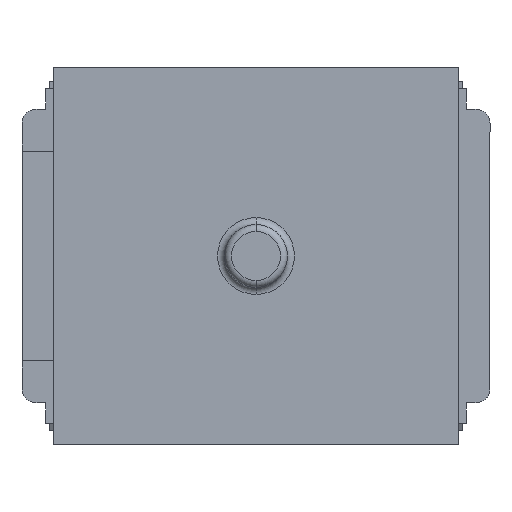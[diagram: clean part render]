
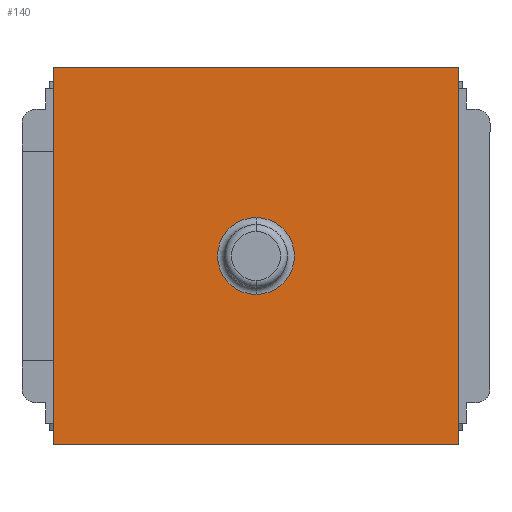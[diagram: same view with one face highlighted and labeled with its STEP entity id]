
A CAD part, front view. The second image highlights one B-rep face of the part: STEP entity #140.
In plain terms, the highlighted planar face has unit normal (0, -1, 0).
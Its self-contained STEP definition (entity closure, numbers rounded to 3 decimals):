
#29 = CARTESIAN_POINT ( 'NONE',  ( -14.5, 0., 13.5 ) ) ;
#38 = VERTEX_POINT ( 'NONE', #10297 ) ;
#67 = DIRECTION ( 'NONE',  ( 0., -1., 0. ) ) ;
#140 = ADVANCED_FACE ( 'NONE', ( #1272, #4230 ), #11520, .T. ) ;
#559 = LINE ( 'NONE', #11567, #11957 ) ;
#809 = LINE ( 'NONE', #8428, #12501 ) ;
#1272 = FACE_OUTER_BOUND ( 'NONE', #3683, .T. ) ;
#1480 = CARTESIAN_POINT ( 'NONE',  ( -14.5, 0., -13.5 ) ) ;
#1670 = DIRECTION ( 'NONE',  ( 0., 0., -1. ) ) ;
#1696 = DIRECTION ( 'NONE',  ( 1., 0., 0. ) ) ;
#2077 = ORIENTED_EDGE ( 'NONE', *, *, #9021, .F. ) ;
#2322 = VERTEX_POINT ( 'NONE', #12895 ) ;
#2893 = DIRECTION ( 'NONE',  ( -1., 0., 0. ) ) ;
#3023 = ORIENTED_EDGE ( 'NONE', *, *, #13638, .F. ) ;
#3104 = CARTESIAN_POINT ( 'NONE',  ( 14.5, 0., -13.5 ) ) ;
#3201 = CARTESIAN_POINT ( 'NONE',  ( 0., 0., 0. ) ) ;
#3608 = DIRECTION ( 'NONE',  ( 0., 1., 0. ) ) ;
#3683 = EDGE_LOOP ( 'NONE', ( #12785, #5862, #3023, #2077 ) ) ;
#4230 = FACE_BOUND ( 'NONE', #7990, .T. ) ;
#4301 = DIRECTION ( 'NONE',  ( 0., 0., 1. ) ) ;
#4398 = ORIENTED_EDGE ( 'NONE', *, *, #6905, .T. ) ;
#5103 = DIRECTION ( 'NONE',  ( 0., 0., 1. ) ) ;
#5650 = CIRCLE ( 'NONE', #9942, 2.75 ) ;
#5862 = ORIENTED_EDGE ( 'NONE', *, *, #6649, .F. ) ;
#6649 = EDGE_CURVE ( 'NONE', #13447, #38, #559, .T. ) ;
#6742 = VECTOR ( 'NONE', #2893, 1000. ) ;
#6905 = EDGE_CURVE ( 'NONE', #7836, #2322, #10182, .T. ) ;
#7040 = ORIENTED_EDGE ( 'NONE', *, *, #11708, .T. ) ;
#7765 = DIRECTION ( 'NONE',  ( 0., 0., -1. ) ) ;
#7836 = VERTEX_POINT ( 'NONE', #13897 ) ;
#7990 = EDGE_LOOP ( 'NONE', ( #4398, #7040 ) ) ;
#8428 = CARTESIAN_POINT ( 'NONE',  ( -14.5, 0., 13.5 ) ) ;
#8449 = AXIS2_PLACEMENT_3D ( 'NONE', #13265, #67, #7765 ) ;
#8809 = VERTEX_POINT ( 'NONE', #3104 ) ;
#9021 = EDGE_CURVE ( 'NONE', #8809, #10496, #9664, .T. ) ;
#9354 = CARTESIAN_POINT ( 'NONE',  ( 14.5, 0., 13.5 ) ) ;
#9465 = LINE ( 'NONE', #9354, #12097 ) ;
#9519 = EDGE_CURVE ( 'NONE', #38, #8809, #9465, .T. ) ;
#9664 = LINE ( 'NONE', #1480, #6742 ) ;
#9942 = AXIS2_PLACEMENT_3D ( 'NONE', #3201, #10889, #4301 ) ;
#9962 = CARTESIAN_POINT ( 'NONE',  ( -14.5, 0., -13.5 ) ) ;
#10182 = CIRCLE ( 'NONE', #13601, 2.75 ) ;
#10183 = CARTESIAN_POINT ( 'NONE',  ( 0., 0., 0. ) ) ;
#10297 = CARTESIAN_POINT ( 'NONE',  ( 14.5, 0., 13.5 ) ) ;
#10496 = VERTEX_POINT ( 'NONE', #9962 ) ;
#10889 = DIRECTION ( 'NONE',  ( 0., 1., 0. ) ) ;
#11308 = DIRECTION ( 'NONE',  ( 0., 0., 1. ) ) ;
#11520 = PLANE ( 'NONE',  #8449 ) ;
#11567 = CARTESIAN_POINT ( 'NONE',  ( -14.5, 0., 13.5 ) ) ;
#11708 = EDGE_CURVE ( 'NONE', #2322, #7836, #5650, .T. ) ;
#11957 = VECTOR ( 'NONE', #1696, 1000. ) ;
#12097 = VECTOR ( 'NONE', #1670, 1000. ) ;
#12501 = VECTOR ( 'NONE', #5103, 1000. ) ;
#12785 = ORIENTED_EDGE ( 'NONE', *, *, #9519, .F. ) ;
#12895 = CARTESIAN_POINT ( 'NONE',  ( 0., 0., 2.75 ) ) ;
#13265 = CARTESIAN_POINT ( 'NONE',  ( 0., 0., 0. ) ) ;
#13447 = VERTEX_POINT ( 'NONE', #29 ) ;
#13601 = AXIS2_PLACEMENT_3D ( 'NONE', #10183, #3608, #11308 ) ;
#13638 = EDGE_CURVE ( 'NONE', #10496, #13447, #809, .T. ) ;
#13897 = CARTESIAN_POINT ( 'NONE',  ( 0., 0., -2.75 ) ) ;
